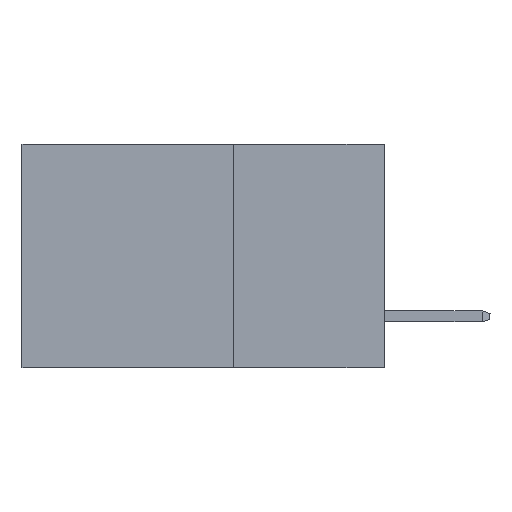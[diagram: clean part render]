
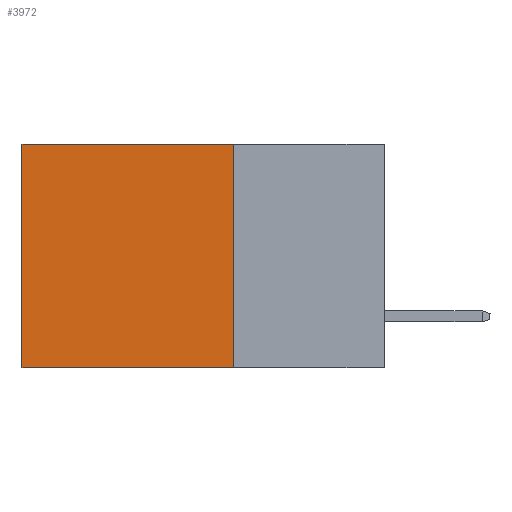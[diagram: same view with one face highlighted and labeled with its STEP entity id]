
A CAD part, left-side view. The second image highlights one B-rep face of the part: STEP entity #3972.
In plain terms, the highlighted planar face has unit normal (-1, 0, 0).
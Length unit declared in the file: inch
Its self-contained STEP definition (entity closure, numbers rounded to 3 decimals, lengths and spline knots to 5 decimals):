
#55 = EDGE_CURVE ( 'NONE', #10116, #5777, #12212, .T. ) ;
#129 = PLANE ( 'NONE',  #13699 ) ;
#309 = VERTEX_POINT ( 'NONE', #2368 ) ;
#799 = ORIENTED_EDGE ( 'NONE', *, *, #7278, .F. ) ;
#2014 = DIRECTION ( 'NONE',  ( 1., 0., 0. ) ) ;
#2210 = LINE ( 'NONE', #9492, #10668 ) ;
#2368 = CARTESIAN_POINT ( 'NONE',  ( 0.2615, 0.25, 0. ) ) ;
#2699 = CARTESIAN_POINT ( 'NONE',  ( 0.2615, 0.6, -0.37 ) ) ;
#3006 = LINE ( 'NONE', #11507, #10356 ) ;
#3265 = EDGE_CURVE ( 'NONE', #309, #10116, #3006, .T. ) ;
#3541 = VERTEX_POINT ( 'NONE', #13480 ) ;
#3833 = ORIENTED_EDGE ( 'NONE', *, *, #3265, .T. ) ;
#3972 = ADVANCED_FACE ( 'NONE', ( #12770 ), #129, .F. ) ;
#5000 = CARTESIAN_POINT ( 'NONE',  ( 0.2615, 0.25, -0.37 ) ) ;
#5097 = EDGE_CURVE ( 'NONE', #309, #3541, #11318, .T. ) ;
#5777 = VERTEX_POINT ( 'NONE', #9898 ) ;
#6027 = DIRECTION ( 'NONE',  ( 0., 1., 0. ) ) ;
#6536 = DIRECTION ( 'NONE',  ( 0., 0., -1. ) ) ;
#6955 = DIRECTION ( 'NONE',  ( 0., 0., -1. ) ) ;
#7278 = EDGE_CURVE ( 'NONE', #3541, #5777, #2210, .T. ) ;
#7403 = ORIENTED_EDGE ( 'NONE', *, *, #5097, .F. ) ;
#8708 = VECTOR ( 'NONE', #6955, 39.37008 ) ;
#9492 = CARTESIAN_POINT ( 'NONE',  ( 0.2615, 0.25, -0.37 ) ) ;
#9569 = ORIENTED_EDGE ( 'NONE', *, *, #55, .T. ) ;
#9898 = CARTESIAN_POINT ( 'NONE',  ( 0.2615, 0.6, -0.37 ) ) ;
#10116 = VERTEX_POINT ( 'NONE', #10853 ) ;
#10356 = VECTOR ( 'NONE', #6027, 39.37008 ) ;
#10668 = VECTOR ( 'NONE', #10671, 39.37008 ) ;
#10671 = DIRECTION ( 'NONE',  ( 0., 1., 0. ) ) ;
#10853 = CARTESIAN_POINT ( 'NONE',  ( 0.2615, 0.6, 0. ) ) ;
#11232 = EDGE_LOOP ( 'NONE', ( #9569, #799, #7403, #3833 ) ) ;
#11318 = LINE ( 'NONE', #5000, #13717 ) ;
#11507 = CARTESIAN_POINT ( 'NONE',  ( 0.2615, 0.25, 0. ) ) ;
#12212 = LINE ( 'NONE', #2699, #8708 ) ;
#12417 = DIRECTION ( 'NONE',  ( 0., 0., -1. ) ) ;
#12649 = CARTESIAN_POINT ( 'NONE',  ( 0.2615, 0.25, -0.37 ) ) ;
#12770 = FACE_OUTER_BOUND ( 'NONE', #11232, .T. ) ;
#13480 = CARTESIAN_POINT ( 'NONE',  ( 0.2615, 0.25, -0.37 ) ) ;
#13699 = AXIS2_PLACEMENT_3D ( 'NONE', #12649, #2014, #6536 ) ;
#13717 = VECTOR ( 'NONE', #12417, 39.37008 ) ;
